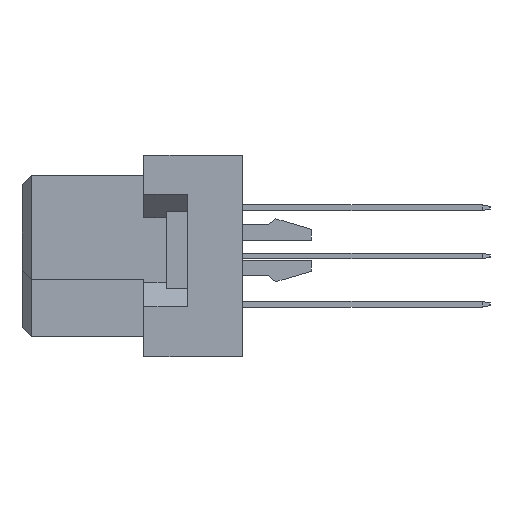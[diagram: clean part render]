
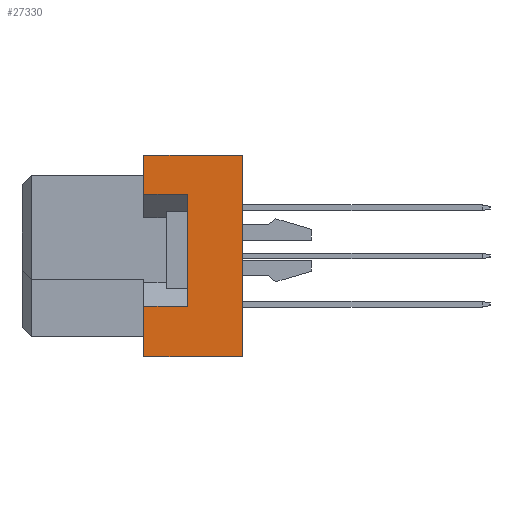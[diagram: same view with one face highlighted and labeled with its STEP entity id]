
A CAD part, left-side view. The second image highlights one B-rep face of the part: STEP entity #27330.
In plain terms, the highlighted planar face has unit normal (-1, 0, 0).
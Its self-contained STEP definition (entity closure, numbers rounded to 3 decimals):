
#1661 = VECTOR ( 'NONE', #2661, 1000. ) ;
#1739 = CARTESIAN_POINT ( 'NONE',  ( -47.5, -6.4, -5.3 ) ) ;
#1825 = VECTOR ( 'NONE', #35991, 1000. ) ;
#2661 = DIRECTION ( 'NONE',  ( 0., 0., 1. ) ) ;
#2696 = EDGE_CURVE ( 'NONE', #26061, #8659, #34001, .T. ) ;
#2973 = EDGE_CURVE ( 'NONE', #26061, #29753, #14796, .T. ) ;
#3499 = CARTESIAN_POINT ( 'NONE',  ( -47.5, -8.7, 3.25 ) ) ;
#4335 = LINE ( 'NONE', #25122, #13149 ) ;
#4781 = LINE ( 'NONE', #1739, #23715 ) ;
#5123 = LINE ( 'NONE', #11380, #30624 ) ;
#5568 = CARTESIAN_POINT ( 'NONE',  ( -47.5, -8.7, 3.25 ) ) ;
#5584 = DIRECTION ( 'NONE',  ( 0., 0., 1. ) ) ;
#5900 = LINE ( 'NONE', #30149, #1661 ) ;
#6353 = DIRECTION ( 'NONE',  ( 0., 1., 0. ) ) ;
#6524 = DIRECTION ( 'NONE',  ( 0., 1., 0. ) ) ;
#8659 = VERTEX_POINT ( 'NONE', #11276 ) ;
#9017 = VERTEX_POINT ( 'NONE', #28793 ) ;
#9266 = LINE ( 'NONE', #11704, #39707 ) ;
#10253 = CARTESIAN_POINT ( 'NONE',  ( -47.5, -11.6, -5.3 ) ) ;
#10684 = CARTESIAN_POINT ( 'NONE',  ( -47.5, -8.7, -2.65 ) ) ;
#11102 = DIRECTION ( 'NONE',  ( 0., 0., 1. ) ) ;
#11276 = CARTESIAN_POINT ( 'NONE',  ( -47.5, -6.4, -5.3 ) ) ;
#11380 = CARTESIAN_POINT ( 'NONE',  ( -47.5, -11.6, 5.3 ) ) ;
#11704 = CARTESIAN_POINT ( 'NONE',  ( -47.5, -6.4, -5.3 ) ) ;
#11802 = VECTOR ( 'NONE', #6353, 1000. ) ;
#11908 = ORIENTED_EDGE ( 'NONE', *, *, #2696, .F. ) ;
#13149 = VECTOR ( 'NONE', #37455, 1000. ) ;
#14437 = ORIENTED_EDGE ( 'NONE', *, *, #21692, .F. ) ;
#14501 = EDGE_CURVE ( 'NONE', #24333, #9017, #4335, .T. ) ;
#14796 = LINE ( 'NONE', #32769, #1825 ) ;
#14988 = VERTEX_POINT ( 'NONE', #32950 ) ;
#16170 = ORIENTED_EDGE ( 'NONE', *, *, #14501, .T. ) ;
#16668 = EDGE_LOOP ( 'NONE', ( #16170, #34364, #11908, #37739, #35711, #35812, #29872, #14437 ) ) ;
#17372 = PLANE ( 'NONE',  #26137 ) ;
#17829 = DIRECTION ( 'NONE',  ( 0., 1., 0. ) ) ;
#19078 = VERTEX_POINT ( 'NONE', #37206 ) ;
#19258 = LINE ( 'NONE', #3499, #11802 ) ;
#19704 = EDGE_CURVE ( 'NONE', #31743, #14988, #19258, .T. ) ;
#20184 = DIRECTION ( 'NONE',  ( -1., 0., 0. ) ) ;
#21692 = EDGE_CURVE ( 'NONE', #24333, #31743, #5900, .T. ) ;
#23409 = CARTESIAN_POINT ( 'NONE',  ( -47.5, -11.6, 5.3 ) ) ;
#23715 = VECTOR ( 'NONE', #5584, 1000. ) ;
#24333 = VERTEX_POINT ( 'NONE', #10684 ) ;
#25122 = CARTESIAN_POINT ( 'NONE',  ( -47.5, -8.7, -2.65 ) ) ;
#26061 = VERTEX_POINT ( 'NONE', #10253 ) ;
#26137 = AXIS2_PLACEMENT_3D ( 'NONE', #23409, #20184, #11102 ) ;
#27240 = DIRECTION ( 'NONE',  ( 0., 0., 1. ) ) ;
#27330 = ADVANCED_FACE ( 'NONE', ( #36150 ), #17372, .T. ) ;
#27475 = EDGE_CURVE ( 'NONE', #14988, #19078, #9266, .T. ) ;
#28119 = CARTESIAN_POINT ( 'NONE',  ( -47.5, -11.6, -5.3 ) ) ;
#28421 = EDGE_CURVE ( 'NONE', #29753, #19078, #5123, .T. ) ;
#28793 = CARTESIAN_POINT ( 'NONE',  ( -47.5, -6.4, -2.65 ) ) ;
#29753 = VERTEX_POINT ( 'NONE', #32998 ) ;
#29872 = ORIENTED_EDGE ( 'NONE', *, *, #19704, .F. ) ;
#30149 = CARTESIAN_POINT ( 'NONE',  ( -47.5, -8.7, -2.65 ) ) ;
#30595 = VECTOR ( 'NONE', #6524, 1000. ) ;
#30624 = VECTOR ( 'NONE', #17829, 1000. ) ;
#31743 = VERTEX_POINT ( 'NONE', #5568 ) ;
#32769 = CARTESIAN_POINT ( 'NONE',  ( -47.5, -11.6, 5.3 ) ) ;
#32950 = CARTESIAN_POINT ( 'NONE',  ( -47.5, -6.4, 3.25 ) ) ;
#32998 = CARTESIAN_POINT ( 'NONE',  ( -47.5, -11.6, 5.3 ) ) ;
#34001 = LINE ( 'NONE', #28119, #30595 ) ;
#34085 = EDGE_CURVE ( 'NONE', #8659, #9017, #4781, .T. ) ;
#34364 = ORIENTED_EDGE ( 'NONE', *, *, #34085, .F. ) ;
#35711 = ORIENTED_EDGE ( 'NONE', *, *, #28421, .T. ) ;
#35812 = ORIENTED_EDGE ( 'NONE', *, *, #27475, .F. ) ;
#35991 = DIRECTION ( 'NONE',  ( 0., 0., 1. ) ) ;
#36150 = FACE_OUTER_BOUND ( 'NONE', #16668, .T. ) ;
#37206 = CARTESIAN_POINT ( 'NONE',  ( -47.5, -6.4, 5.3 ) ) ;
#37455 = DIRECTION ( 'NONE',  ( 0., 1., 0. ) ) ;
#37739 = ORIENTED_EDGE ( 'NONE', *, *, #2973, .T. ) ;
#39707 = VECTOR ( 'NONE', #27240, 1000. ) ;
